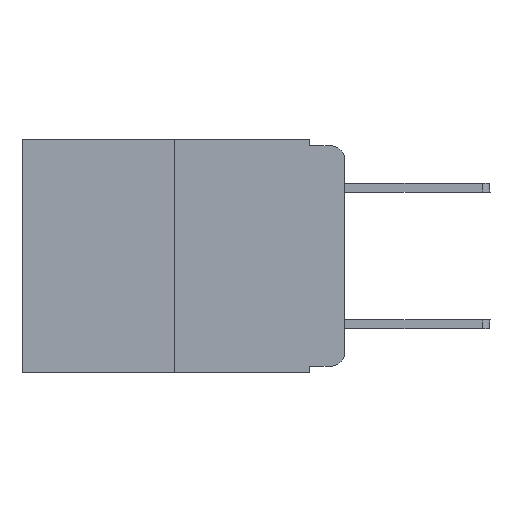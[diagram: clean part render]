
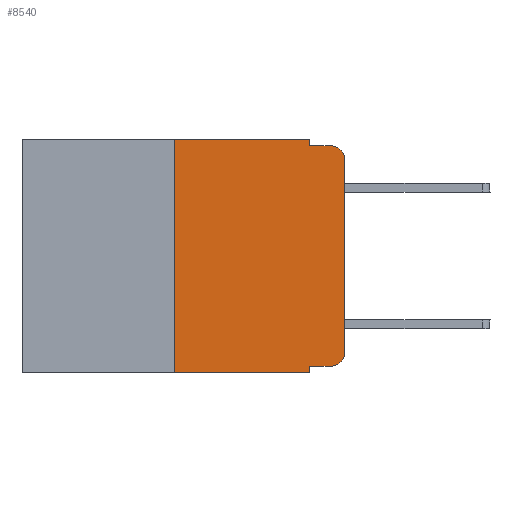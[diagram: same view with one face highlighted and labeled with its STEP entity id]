
A CAD part, left-side view. The second image highlights one B-rep face of the part: STEP entity #8540.
In plain terms, the highlighted planar face has unit normal (-1, 0, 0).
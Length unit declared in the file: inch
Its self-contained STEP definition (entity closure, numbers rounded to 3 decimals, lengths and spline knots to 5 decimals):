
#64 = CARTESIAN_POINT ( 'NONE',  ( 0., 0.02, -0.313 ) ) ;
#66 = CARTESIAN_POINT ( 'NONE',  ( 0., 0.473, -0.343 ) ) ;
#409 = VERTEX_POINT ( 'NONE', #1092 ) ;
#452 = LINE ( 'NONE', #13904, #6963 ) ;
#655 = EDGE_LOOP ( 'NONE', ( #11751, #11790, #14026, #1454, #12336, #11250, #1070, #832, #13201, #8132 ) ) ;
#832 = ORIENTED_EDGE ( 'NONE', *, *, #3093, .F. ) ;
#1026 = FACE_OUTER_BOUND ( 'NONE', #655, .T. ) ;
#1070 = ORIENTED_EDGE ( 'NONE', *, *, #8491, .T. ) ;
#1092 = CARTESIAN_POINT ( 'NONE',  ( 0., 0.25, 0. ) ) ;
#1221 = AXIS2_PLACEMENT_3D ( 'NONE', #10178, #14709, #4479 ) ;
#1256 = DIRECTION ( 'NONE',  ( 0., 0., -1. ) ) ;
#1346 = VERTEX_POINT ( 'NONE', #13782 ) ;
#1368 = VERTEX_POINT ( 'NONE', #14147 ) ;
#1454 = ORIENTED_EDGE ( 'NONE', *, *, #5708, .F. ) ;
#1525 = DIRECTION ( 'NONE',  ( 0., 0., -1. ) ) ;
#1655 = EDGE_CURVE ( 'NONE', #14640, #6579, #7733, .T. ) ;
#1658 = CARTESIAN_POINT ( 'NONE',  ( 0., 0., -0.313 ) ) ;
#1988 = CARTESIAN_POINT ( 'NONE',  ( 0., 0.051, -0.333 ) ) ;
#2186 = VECTOR ( 'NONE', #12223, 39.37008 ) ;
#2391 = CARTESIAN_POINT ( 'NONE',  ( 0., 0.02, -0.03 ) ) ;
#2908 = CARTESIAN_POINT ( 'NONE',  ( 0., 0.051, -0.343 ) ) ;
#3093 = EDGE_CURVE ( 'NONE', #3725, #4311, #7885, .T. ) ;
#3205 = CARTESIAN_POINT ( 'NONE',  ( 0., 0.25, -0.343 ) ) ;
#3568 = DIRECTION ( 'NONE',  ( -1., 0., 0. ) ) ;
#3586 = DIRECTION ( 'NONE',  ( 0., -1., 0. ) ) ;
#3725 = VERTEX_POINT ( 'NONE', #1988 ) ;
#4149 = EDGE_CURVE ( 'NONE', #6579, #4540, #12843, .T. ) ;
#4266 = VECTOR ( 'NONE', #1525, 39.37008 ) ;
#4311 = VERTEX_POINT ( 'NONE', #2908 ) ;
#4345 = LINE ( 'NONE', #10349, #13499 ) ;
#4440 = VERTEX_POINT ( 'NONE', #3205 ) ;
#4479 = DIRECTION ( 'NONE',  ( 0., 0., -1. ) ) ;
#4496 = DIRECTION ( 'NONE',  ( 0., 0., -1. ) ) ;
#4540 = VERTEX_POINT ( 'NONE', #4678 ) ;
#4678 = CARTESIAN_POINT ( 'NONE',  ( 0., 0.02, -0.01 ) ) ;
#5555 = DIRECTION ( 'NONE',  ( 0., -1., 0. ) ) ;
#5605 = PLANE ( 'NONE',  #1221 ) ;
#5708 = EDGE_CURVE ( 'NONE', #14080, #1346, #11627, .T. ) ;
#6106 = CARTESIAN_POINT ( 'NONE',  ( 0., 0.051, 0. ) ) ;
#6579 = VERTEX_POINT ( 'NONE', #9838 ) ;
#6600 = CARTESIAN_POINT ( 'NONE',  ( 0., 0., 0. ) ) ;
#6963 = VECTOR ( 'NONE', #3586, 39.37008 ) ;
#7645 = EDGE_CURVE ( 'NONE', #1368, #14640, #11019, .T. ) ;
#7733 = LINE ( 'NONE', #6600, #11126 ) ;
#7807 = EDGE_CURVE ( 'NONE', #4440, #409, #11113, .T. ) ;
#7885 = LINE ( 'NONE', #14731, #9250 ) ;
#7938 = DIRECTION ( 'NONE',  ( 0., 0., -1. ) ) ;
#7942 = LINE ( 'NONE', #66, #14319 ) ;
#7999 = CARTESIAN_POINT ( 'NONE',  ( 0., 0.051, 0. ) ) ;
#8132 = ORIENTED_EDGE ( 'NONE', *, *, #7645, .T. ) ;
#8170 = AXIS2_PLACEMENT_3D ( 'NONE', #64, #3568, #7938 ) ;
#8491 = EDGE_CURVE ( 'NONE', #4440, #4311, #7942, .T. ) ;
#8540 = ADVANCED_FACE ( 'NONE', ( #1026 ), #5605, .F. ) ;
#8979 = EDGE_CURVE ( 'NONE', #409, #14080, #12257, .T. ) ;
#9175 = EDGE_CURVE ( 'NONE', #1346, #4540, #452, .T. ) ;
#9250 = VECTOR ( 'NONE', #4496, 39.37008 ) ;
#9838 = CARTESIAN_POINT ( 'NONE',  ( 0., 0., -0.03 ) ) ;
#10105 = DIRECTION ( 'NONE',  ( 0., -1., 0. ) ) ;
#10178 = CARTESIAN_POINT ( 'NONE',  ( 0., 0.473, 0. ) ) ;
#10349 = CARTESIAN_POINT ( 'NONE',  ( 0., 0.051, -0.333 ) ) ;
#10993 = VECTOR ( 'NONE', #12183, 39.37008 ) ;
#11019 = CIRCLE ( 'NONE', #8170, 0.02 ) ;
#11113 = LINE ( 'NONE', #12151, #2186 ) ;
#11126 = VECTOR ( 'NONE', #11152, 39.37008 ) ;
#11152 = DIRECTION ( 'NONE',  ( 0., 0., 1. ) ) ;
#11250 = ORIENTED_EDGE ( 'NONE', *, *, #7807, .F. ) ;
#11627 = LINE ( 'NONE', #6106, #4266 ) ;
#11751 = ORIENTED_EDGE ( 'NONE', *, *, #1655, .T. ) ;
#11790 = ORIENTED_EDGE ( 'NONE', *, *, #4149, .T. ) ;
#12151 = CARTESIAN_POINT ( 'NONE',  ( 0., 0.25, 0. ) ) ;
#12183 = DIRECTION ( 'NONE',  ( 0., -1., 0. ) ) ;
#12223 = DIRECTION ( 'NONE',  ( 0., 0., 1. ) ) ;
#12257 = LINE ( 'NONE', #13313, #10993 ) ;
#12336 = ORIENTED_EDGE ( 'NONE', *, *, #8979, .F. ) ;
#12768 = DIRECTION ( 'NONE',  ( -1., 0., 0. ) ) ;
#12843 = CIRCLE ( 'NONE', #13074, 0.02 ) ;
#13074 = AXIS2_PLACEMENT_3D ( 'NONE', #2391, #12768, #1256 ) ;
#13201 = ORIENTED_EDGE ( 'NONE', *, *, #13539, .T. ) ;
#13313 = CARTESIAN_POINT ( 'NONE',  ( 0., 0.473, 0. ) ) ;
#13499 = VECTOR ( 'NONE', #5555, 39.37008 ) ;
#13539 = EDGE_CURVE ( 'NONE', #3725, #1368, #4345, .T. ) ;
#13782 = CARTESIAN_POINT ( 'NONE',  ( 0., 0.051, -0.01 ) ) ;
#13904 = CARTESIAN_POINT ( 'NONE',  ( 0., 0.051, -0.01 ) ) ;
#14026 = ORIENTED_EDGE ( 'NONE', *, *, #9175, .F. ) ;
#14080 = VERTEX_POINT ( 'NONE', #7999 ) ;
#14147 = CARTESIAN_POINT ( 'NONE',  ( 0., 0.02, -0.333 ) ) ;
#14319 = VECTOR ( 'NONE', #10105, 39.37008 ) ;
#14640 = VERTEX_POINT ( 'NONE', #1658 ) ;
#14709 = DIRECTION ( 'NONE',  ( 1., 0., 0. ) ) ;
#14731 = CARTESIAN_POINT ( 'NONE',  ( 0., 0.051, 0. ) ) ;
